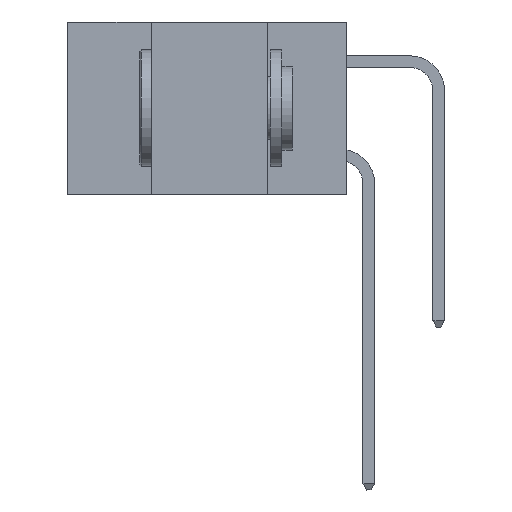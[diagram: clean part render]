
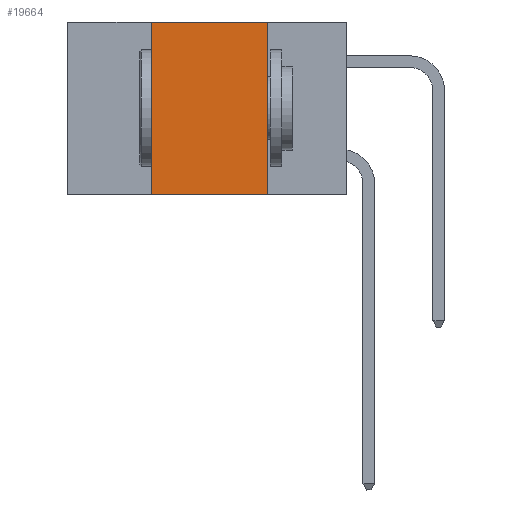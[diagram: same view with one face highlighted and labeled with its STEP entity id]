
A CAD part, left-side view. The second image highlights one B-rep face of the part: STEP entity #19664.
In plain terms, the highlighted planar face has unit normal (-1, 0, 0).
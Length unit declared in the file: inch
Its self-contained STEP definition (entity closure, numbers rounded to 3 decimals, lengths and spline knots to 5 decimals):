
#119 = DIRECTION ( 'NONE',  ( 0., 0., -1. ) ) ;
#1814 = VECTOR ( 'NONE', #24070, 39.37008 ) ;
#6257 = EDGE_CURVE ( 'NONE', #32821, #10334, #27397, .T. ) ;
#7961 = CARTESIAN_POINT ( 'NONE',  ( 0., 0.6, 0. ) ) ;
#8677 = CARTESIAN_POINT ( 'NONE',  ( 0., 0.6, 0. ) ) ;
#8940 = ORIENTED_EDGE ( 'NONE', *, *, #24963, .T. ) ;
#10334 = VERTEX_POINT ( 'NONE', #27944 ) ;
#12011 = VERTEX_POINT ( 'NONE', #31466 ) ;
#12595 = VECTOR ( 'NONE', #18968, 39.37008 ) ;
#14217 = CARTESIAN_POINT ( 'NONE',  ( 0., 0.17, -0.37 ) ) ;
#14443 = PLANE ( 'NONE',  #27429 ) ;
#15961 = EDGE_CURVE ( 'NONE', #12011, #28645, #24175, .T. ) ;
#17671 = DIRECTION ( 'NONE',  ( 1., 0., 0. ) ) ;
#18690 = CARTESIAN_POINT ( 'NONE',  ( 0., 0.42, -0.37 ) ) ;
#18968 = DIRECTION ( 'NONE',  ( 0., -1., 0. ) ) ;
#19146 = EDGE_CURVE ( 'NONE', #10334, #12011, #20019, .T. ) ;
#19664 = ADVANCED_FACE ( 'NONE', ( #25372 ), #14443, .F. ) ;
#20019 = LINE ( 'NONE', #8677, #35706 ) ;
#22705 = CARTESIAN_POINT ( 'NONE',  ( 0., 0.17, 0. ) ) ;
#22931 = ORIENTED_EDGE ( 'NONE', *, *, #15961, .F. ) ;
#24070 = DIRECTION ( 'NONE',  ( 0., 0., 1. ) ) ;
#24175 = LINE ( 'NONE', #22705, #38913 ) ;
#24963 = EDGE_CURVE ( 'NONE', #32821, #28645, #29387, .T. ) ;
#25372 = FACE_OUTER_BOUND ( 'NONE', #39183, .T. ) ;
#27068 = CARTESIAN_POINT ( 'NONE',  ( 0., 0.42, 0. ) ) ;
#27397 = LINE ( 'NONE', #27068, #1814 ) ;
#27429 = AXIS2_PLACEMENT_3D ( 'NONE', #7961, #17671, #39667 ) ;
#27944 = CARTESIAN_POINT ( 'NONE',  ( 0., 0.42, 0. ) ) ;
#28645 = VERTEX_POINT ( 'NONE', #14217 ) ;
#29387 = LINE ( 'NONE', #34561, #12595 ) ;
#31466 = CARTESIAN_POINT ( 'NONE',  ( 0., 0.17, 0. ) ) ;
#32206 = ORIENTED_EDGE ( 'NONE', *, *, #19146, .F. ) ;
#32821 = VERTEX_POINT ( 'NONE', #18690 ) ;
#33197 = ORIENTED_EDGE ( 'NONE', *, *, #6257, .F. ) ;
#34561 = CARTESIAN_POINT ( 'NONE',  ( 0., 0.6, -0.37 ) ) ;
#35706 = VECTOR ( 'NONE', #40380, 39.37008 ) ;
#38913 = VECTOR ( 'NONE', #119, 39.37008 ) ;
#39183 = EDGE_LOOP ( 'NONE', ( #22931, #32206, #33197, #8940 ) ) ;
#39667 = DIRECTION ( 'NONE',  ( 0., 0., -1. ) ) ;
#40380 = DIRECTION ( 'NONE',  ( 0., -1., 0. ) ) ;
